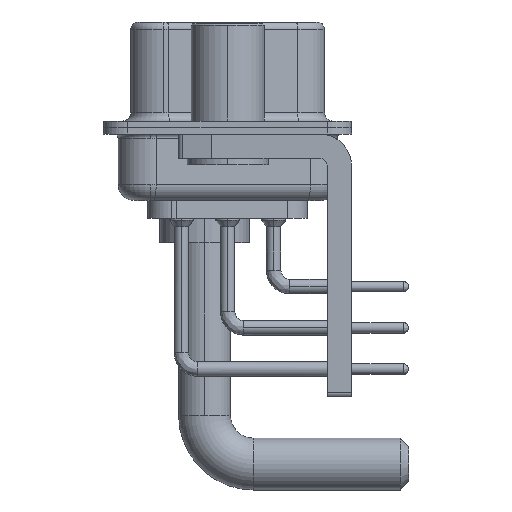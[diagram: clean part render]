
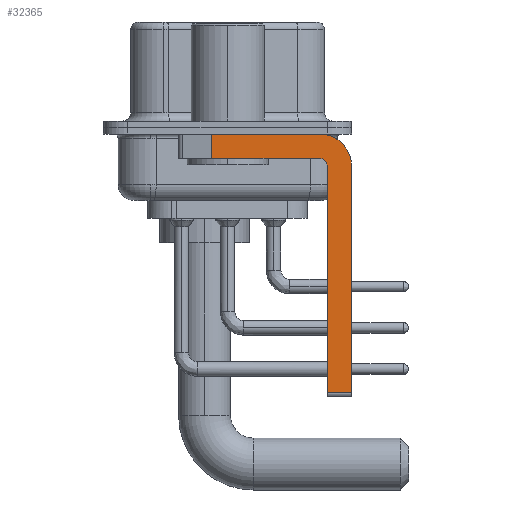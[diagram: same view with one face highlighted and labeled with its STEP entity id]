
A CAD part, left-side view. The second image highlights one B-rep face of the part: STEP entity #32365.
In plain terms, the highlighted planar face has unit normal (-1, 0, 0).
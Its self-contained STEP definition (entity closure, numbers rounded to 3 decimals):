
#2251 = FACE_OUTER_BOUND ( 'NONE', #21327, .T. ) ;
#3025 = CARTESIAN_POINT ( 'NONE',  ( -2.9, 0.978, -0.4 ) ) ;
#3216 = CARTESIAN_POINT ( 'NONE',  ( -2.9, 0.978, -1.9 ) ) ;
#3303 = CARTESIAN_POINT ( 'NONE',  ( -2.9, -6.15, -16.6 ) ) ;
#3824 = LINE ( 'NONE', #3216, #20630 ) ;
#4886 = EDGE_CURVE ( 'NONE', #17954, #17276, #8211, .T. ) ;
#5480 = PLANE ( 'NONE',  #10035 ) ;
#5599 = VECTOR ( 'NONE', #6421, 1000. ) ;
#6421 = DIRECTION ( 'NONE',  ( 0., -1., 0. ) ) ;
#6589 = ORIENTED_EDGE ( 'NONE', *, *, #4886, .F. ) ;
#6714 = CARTESIAN_POINT ( 'NONE',  ( -2.9, -7.65, -2.4 ) ) ;
#8121 = CARTESIAN_POINT ( 'NONE',  ( -2.9, 0.978, -1.9 ) ) ;
#8152 = EDGE_CURVE ( 'NONE', #10901, #24434, #3824, .T. ) ;
#8155 = CARTESIAN_POINT ( 'NONE',  ( -2.9, -5.65, -0.4 ) ) ;
#8195 = VECTOR ( 'NONE', #22453, 1000. ) ;
#8206 = ORIENTED_EDGE ( 'NONE', *, *, #36377, .F. ) ;
#8211 = CIRCLE ( 'NONE', #25676, 0.5 ) ;
#8261 = CARTESIAN_POINT ( 'NONE',  ( -2.9, -7.65, -2.4 ) ) ;
#8481 = DIRECTION ( 'NONE',  ( 1., 0., 0. ) ) ;
#8878 = CIRCLE ( 'NONE', #31517, 2. ) ;
#8985 = VERTEX_POINT ( 'NONE', #36439 ) ;
#9799 = VECTOR ( 'NONE', #11698, 1000. ) ;
#9920 = DIRECTION ( 'NONE',  ( 0., -1., 0. ) ) ;
#10035 = AXIS2_PLACEMENT_3D ( 'NONE', #36373, #8481, #14560 ) ;
#10901 = VERTEX_POINT ( 'NONE', #3025 ) ;
#11493 = ORIENTED_EDGE ( 'NONE', *, *, #27070, .F. ) ;
#11698 = DIRECTION ( 'NONE',  ( 0., 0., -1. ) ) ;
#12156 = DIRECTION ( 'NONE',  ( 1., 0., 0. ) ) ;
#12501 = CARTESIAN_POINT ( 'NONE',  ( -2.9, 3., -0.4 ) ) ;
#14396 = ORIENTED_EDGE ( 'NONE', *, *, #25026, .F. ) ;
#14537 = LINE ( 'NONE', #8261, #9799 ) ;
#14560 = DIRECTION ( 'NONE',  ( 0., 0., -1. ) ) ;
#17276 = VERTEX_POINT ( 'NONE', #20722 ) ;
#17898 = VECTOR ( 'NONE', #9920, 1000. ) ;
#17954 = VERTEX_POINT ( 'NONE', #31031 ) ;
#18442 = VERTEX_POINT ( 'NONE', #6714 ) ;
#18891 = ORIENTED_EDGE ( 'NONE', *, *, #34586, .T. ) ;
#19042 = LINE ( 'NONE', #31372, #17898 ) ;
#20398 = ORIENTED_EDGE ( 'NONE', *, *, #25416, .F. ) ;
#20450 = CARTESIAN_POINT ( 'NONE',  ( -2.9, -5.65, -2.4 ) ) ;
#20630 = VECTOR ( 'NONE', #28075, 1000. ) ;
#20652 = DIRECTION ( 'NONE',  ( 0., 0., 1. ) ) ;
#20722 = CARTESIAN_POINT ( 'NONE',  ( -2.9, -5.65, -1.9 ) ) ;
#21270 = DIRECTION ( 'NONE',  ( 0., 0., 1. ) ) ;
#21327 = EDGE_LOOP ( 'NONE', ( #14396, #36672, #20398, #6589, #27660, #18891, #11493, #8206 ) ) ;
#22453 = DIRECTION ( 'NONE',  ( 0., 1., 0. ) ) ;
#22680 = VERTEX_POINT ( 'NONE', #8155 ) ;
#24296 = DIRECTION ( 'NONE',  ( 0., 0., -1. ) ) ;
#24434 = VERTEX_POINT ( 'NONE', #8121 ) ;
#25026 = EDGE_CURVE ( 'NONE', #10901, #22680, #34713, .T. ) ;
#25416 = EDGE_CURVE ( 'NONE', #17276, #24434, #25494, .T. ) ;
#25494 = LINE ( 'NONE', #35166, #8195 ) ;
#25676 = AXIS2_PLACEMENT_3D ( 'NONE', #20450, #32578, #20652 ) ;
#27070 = EDGE_CURVE ( 'NONE', #18442, #8985, #14537, .T. ) ;
#27660 = ORIENTED_EDGE ( 'NONE', *, *, #31189, .F. ) ;
#28075 = DIRECTION ( 'NONE',  ( 0., 0., -1. ) ) ;
#28810 = VERTEX_POINT ( 'NONE', #30862 ) ;
#29350 = VECTOR ( 'NONE', #21270, 1000. ) ;
#30862 = CARTESIAN_POINT ( 'NONE',  ( -2.9, -6.15, -16.35 ) ) ;
#31031 = CARTESIAN_POINT ( 'NONE',  ( -2.9, -6.15, -2.4 ) ) ;
#31189 = EDGE_CURVE ( 'NONE', #28810, #17954, #36016, .T. ) ;
#31372 = CARTESIAN_POINT ( 'NONE',  ( -2.9, -5.65, -16.35 ) ) ;
#31517 = AXIS2_PLACEMENT_3D ( 'NONE', #39631, #12156, #24296 ) ;
#32365 = ADVANCED_FACE ( 'NONE', ( #2251 ), #5480, .F. ) ;
#32578 = DIRECTION ( 'NONE',  ( -1., 0., 0. ) ) ;
#34586 = EDGE_CURVE ( 'NONE', #28810, #8985, #19042, .T. ) ;
#34713 = LINE ( 'NONE', #12501, #5599 ) ;
#35166 = CARTESIAN_POINT ( 'NONE',  ( -2.9, -5.65, -1.9 ) ) ;
#36016 = LINE ( 'NONE', #3303, #29350 ) ;
#36373 = CARTESIAN_POINT ( 'NONE',  ( -2.9, -5.65, -2.4 ) ) ;
#36377 = EDGE_CURVE ( 'NONE', #22680, #18442, #8878, .T. ) ;
#36439 = CARTESIAN_POINT ( 'NONE',  ( -2.9, -7.65, -16.35 ) ) ;
#36672 = ORIENTED_EDGE ( 'NONE', *, *, #8152, .T. ) ;
#39631 = CARTESIAN_POINT ( 'NONE',  ( -2.9, -5.65, -2.4 ) ) ;
